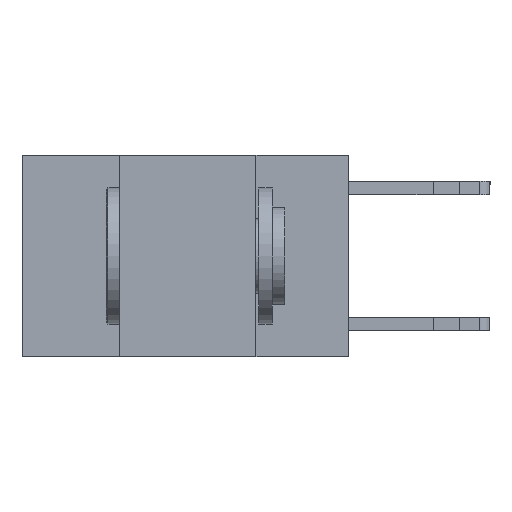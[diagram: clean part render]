
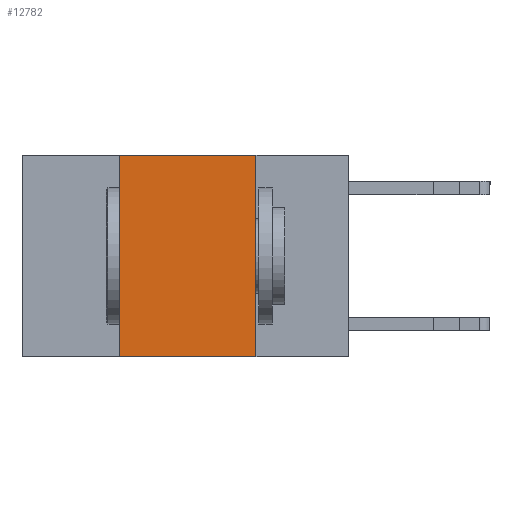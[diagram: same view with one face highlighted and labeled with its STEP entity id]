
A CAD part, left-side view. The second image highlights one B-rep face of the part: STEP entity #12782.
In plain terms, the highlighted planar face has unit normal (-1, 0, 0).
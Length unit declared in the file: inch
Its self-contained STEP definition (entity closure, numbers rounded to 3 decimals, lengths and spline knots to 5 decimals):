
#149 = EDGE_CURVE ( 'NONE', #23156, #307, #9399, .T. ) ;
#307 = VERTEX_POINT ( 'NONE', #945 ) ;
#508 = VECTOR ( 'NONE', #15292, 39.37008 ) ;
#945 = CARTESIAN_POINT ( 'NONE',  ( 0., 0.42, 0. ) ) ;
#956 = VERTEX_POINT ( 'NONE', #9081 ) ;
#1028 = CARTESIAN_POINT ( 'NONE',  ( 0., 0.6, -0.37 ) ) ;
#1261 = VECTOR ( 'NONE', #21018, 39.37008 ) ;
#3673 = PLANE ( 'NONE',  #17095 ) ;
#3900 = DIRECTION ( 'NONE',  ( 1., 0., 0. ) ) ;
#5443 = FACE_OUTER_BOUND ( 'NONE', #18929, .T. ) ;
#7317 = ORIENTED_EDGE ( 'NONE', *, *, #16095, .F. ) ;
#8021 = EDGE_CURVE ( 'NONE', #23156, #956, #10057, .T. ) ;
#8295 = LINE ( 'NONE', #22894, #9075 ) ;
#8517 = CARTESIAN_POINT ( 'NONE',  ( 0., 0.42, -0.37 ) ) ;
#9040 = DIRECTION ( 'NONE',  ( 0., 0., 1. ) ) ;
#9075 = VECTOR ( 'NONE', #13863, 39.37008 ) ;
#9081 = CARTESIAN_POINT ( 'NONE',  ( 0., 0.17, -0.37 ) ) ;
#9399 = LINE ( 'NONE', #18167, #21732 ) ;
#9505 = EDGE_CURVE ( 'NONE', #307, #17389, #8295, .T. ) ;
#10057 = LINE ( 'NONE', #1028, #508 ) ;
#10909 = CARTESIAN_POINT ( 'NONE',  ( 0., 0.6, 0. ) ) ;
#11764 = LINE ( 'NONE', #19340, #1261 ) ;
#12782 = ADVANCED_FACE ( 'NONE', ( #5443 ), #3673, .F. ) ;
#13193 = ORIENTED_EDGE ( 'NONE', *, *, #9505, .F. ) ;
#13863 = DIRECTION ( 'NONE',  ( 0., -1., 0. ) ) ;
#13993 = ORIENTED_EDGE ( 'NONE', *, *, #8021, .T. ) ;
#15292 = DIRECTION ( 'NONE',  ( 0., -1., 0. ) ) ;
#16095 = EDGE_CURVE ( 'NONE', #17389, #956, #11764, .T. ) ;
#17095 = AXIS2_PLACEMENT_3D ( 'NONE', #10909, #3900, #18137 ) ;
#17389 = VERTEX_POINT ( 'NONE', #22234 ) ;
#17612 = ORIENTED_EDGE ( 'NONE', *, *, #149, .F. ) ;
#18137 = DIRECTION ( 'NONE',  ( 0., 0., -1. ) ) ;
#18167 = CARTESIAN_POINT ( 'NONE',  ( 0., 0.42, 0. ) ) ;
#18929 = EDGE_LOOP ( 'NONE', ( #7317, #13193, #17612, #13993 ) ) ;
#19340 = CARTESIAN_POINT ( 'NONE',  ( 0., 0.17, 0. ) ) ;
#21018 = DIRECTION ( 'NONE',  ( 0., 0., -1. ) ) ;
#21732 = VECTOR ( 'NONE', #9040, 39.37008 ) ;
#22234 = CARTESIAN_POINT ( 'NONE',  ( 0., 0.17, 0. ) ) ;
#22894 = CARTESIAN_POINT ( 'NONE',  ( 0., 0.6, 0. ) ) ;
#23156 = VERTEX_POINT ( 'NONE', #8517 ) ;
